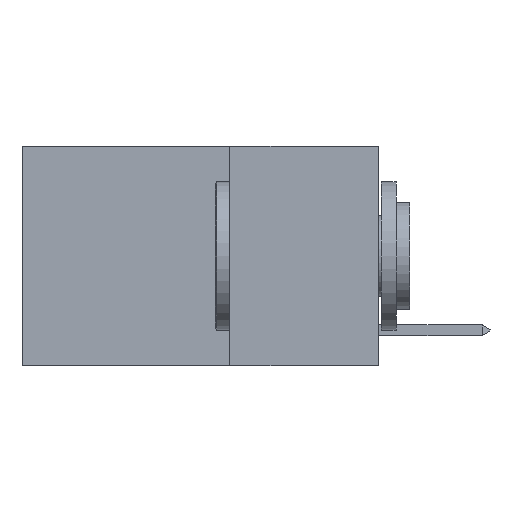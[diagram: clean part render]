
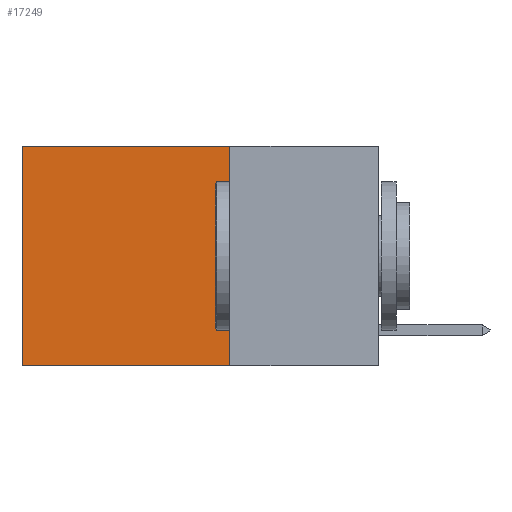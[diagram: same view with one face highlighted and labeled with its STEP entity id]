
A CAD part, left-side view. The second image highlights one B-rep face of the part: STEP entity #17249.
In plain terms, the highlighted planar face has unit normal (-1, 0, 0).
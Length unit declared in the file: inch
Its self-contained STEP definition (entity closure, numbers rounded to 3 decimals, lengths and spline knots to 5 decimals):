
#45 = VECTOR ( 'NONE', #19625, 39.37008 ) ;
#920 = CARTESIAN_POINT ( 'NONE',  ( 0.2625, 0.6, 0. ) ) ;
#1461 = LINE ( 'NONE', #15833, #17944 ) ;
#1707 = ORIENTED_EDGE ( 'NONE', *, *, #22605, .F. ) ;
#2369 = VERTEX_POINT ( 'NONE', #920 ) ;
#4108 = FACE_OUTER_BOUND ( 'NONE', #10079, .T. ) ;
#4419 = EDGE_CURVE ( 'NONE', #17179, #13856, #1461, .T. ) ;
#4577 = ORIENTED_EDGE ( 'NONE', *, *, #4419, .F. ) ;
#4810 = VECTOR ( 'NONE', #15818, 39.37008 ) ;
#5274 = ORIENTED_EDGE ( 'NONE', *, *, #10807, .T. ) ;
#5786 = CARTESIAN_POINT ( 'NONE',  ( 0.2625, 0.25, 0. ) ) ;
#7475 = VECTOR ( 'NONE', #19740, 39.37008 ) ;
#8821 = DIRECTION ( 'NONE',  ( 0., 0., -1. ) ) ;
#10079 = EDGE_LOOP ( 'NONE', ( #5274, #1707, #4577, #18738 ) ) ;
#10133 = LINE ( 'NONE', #15579, #4810 ) ;
#10807 = EDGE_CURVE ( 'NONE', #2369, #11327, #17683, .T. ) ;
#11327 = VERTEX_POINT ( 'NONE', #23792 ) ;
#11452 = DIRECTION ( 'NONE',  ( 1., 0., 0. ) ) ;
#11562 = PLANE ( 'NONE',  #23212 ) ;
#12668 = CARTESIAN_POINT ( 'NONE',  ( 0.2625, 0.25, -0.37 ) ) ;
#13856 = VERTEX_POINT ( 'NONE', #22649 ) ;
#14576 = CARTESIAN_POINT ( 'NONE',  ( 0.2625, 0.25, 0. ) ) ;
#15051 = DIRECTION ( 'NONE',  ( 0., 0., -1. ) ) ;
#15579 = CARTESIAN_POINT ( 'NONE',  ( 0.2625, 0.25, 0. ) ) ;
#15818 = DIRECTION ( 'NONE',  ( 0., 1., 0. ) ) ;
#15833 = CARTESIAN_POINT ( 'NONE',  ( 0.2625, 0.25, 0. ) ) ;
#16423 = LINE ( 'NONE', #12668, #7475 ) ;
#17179 = VERTEX_POINT ( 'NONE', #14576 ) ;
#17249 = ADVANCED_FACE ( 'NONE', ( #4108 ), #11562, .F. ) ;
#17683 = LINE ( 'NONE', #23337, #45 ) ;
#17944 = VECTOR ( 'NONE', #8821, 39.37008 ) ;
#18738 = ORIENTED_EDGE ( 'NONE', *, *, #22532, .T. ) ;
#19625 = DIRECTION ( 'NONE',  ( 0., 0., -1. ) ) ;
#19740 = DIRECTION ( 'NONE',  ( 0., 1., 0. ) ) ;
#22532 = EDGE_CURVE ( 'NONE', #17179, #2369, #10133, .T. ) ;
#22605 = EDGE_CURVE ( 'NONE', #13856, #11327, #16423, .T. ) ;
#22649 = CARTESIAN_POINT ( 'NONE',  ( 0.2625, 0.25, -0.37 ) ) ;
#23212 = AXIS2_PLACEMENT_3D ( 'NONE', #5786, #11452, #15051 ) ;
#23337 = CARTESIAN_POINT ( 'NONE',  ( 0.2625, 0.6, 0. ) ) ;
#23792 = CARTESIAN_POINT ( 'NONE',  ( 0.2625, 0.6, -0.37 ) ) ;
